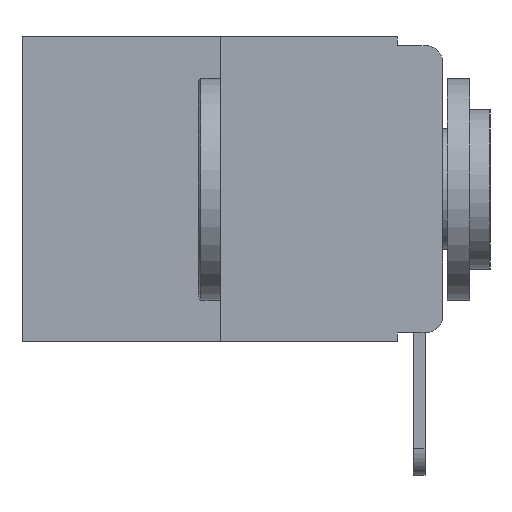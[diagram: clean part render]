
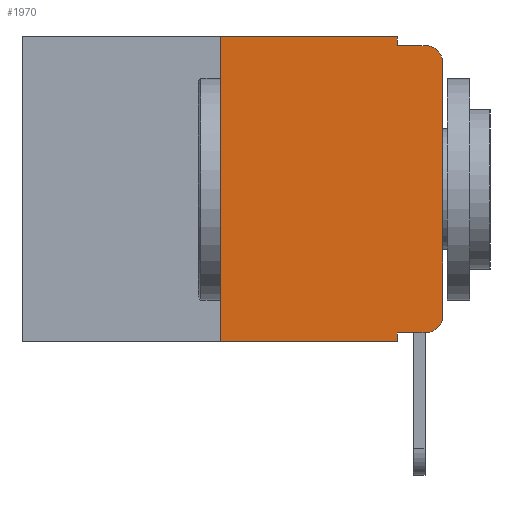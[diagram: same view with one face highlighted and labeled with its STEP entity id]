
A CAD part, left-side view. The second image highlights one B-rep face of the part: STEP entity #1970.
In plain terms, the highlighted planar face has unit normal (-1, 0, 0).
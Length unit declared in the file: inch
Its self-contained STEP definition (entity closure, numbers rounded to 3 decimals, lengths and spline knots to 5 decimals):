
#492 = CARTESIAN_POINT ( 'NONE',  ( 0., 0.051, -0.343 ) ) ;
#544 = VECTOR ( 'NONE', #5614, 39.37008 ) ;
#664 = FACE_OUTER_BOUND ( 'NONE', #9683, .T. ) ;
#940 = CARTESIAN_POINT ( 'NONE',  ( 0., 0.25, -0.343 ) ) ;
#1125 = VERTEX_POINT ( 'NONE', #9532 ) ;
#1679 = EDGE_CURVE ( 'NONE', #8181, #10054, #12038, .T. ) ;
#1754 = EDGE_CURVE ( 'NONE', #8181, #7487, #8797, .T. ) ;
#1970 = ADVANCED_FACE ( 'NONE', ( #664 ), #5951, .F. ) ;
#2189 = VERTEX_POINT ( 'NONE', #2217 ) ;
#2217 = CARTESIAN_POINT ( 'NONE',  ( 0., 0.02, -0.333 ) ) ;
#2447 = AXIS2_PLACEMENT_3D ( 'NONE', #4234, #10577, #5188 ) ;
#2629 = ORIENTED_EDGE ( 'NONE', *, *, #6933, .F. ) ;
#3120 = ORIENTED_EDGE ( 'NONE', *, *, #8857, .F. ) ;
#3358 = CARTESIAN_POINT ( 'NONE',  ( 0., 0.25, 0. ) ) ;
#3360 = LINE ( 'NONE', #7382, #544 ) ;
#3364 = CARTESIAN_POINT ( 'NONE',  ( 0., 0., -0.313 ) ) ;
#3394 = DIRECTION ( 'NONE',  ( 0., 0., 1. ) ) ;
#3437 = CIRCLE ( 'NONE', #7698, 0.02 ) ;
#3554 = LINE ( 'NONE', #5268, #8152 ) ;
#3770 = ORIENTED_EDGE ( 'NONE', *, *, #7630, .T. ) ;
#4046 = ORIENTED_EDGE ( 'NONE', *, *, #10227, .F. ) ;
#4164 = VECTOR ( 'NONE', #11022, 39.37008 ) ;
#4171 = CARTESIAN_POINT ( 'NONE',  ( 0., 0.051, -0.333 ) ) ;
#4234 = CARTESIAN_POINT ( 'NONE',  ( 0., 0.02, -0.03 ) ) ;
#4298 = CARTESIAN_POINT ( 'NONE',  ( 0., 0.051, -0.333 ) ) ;
#4332 = DIRECTION ( 'NONE',  ( 0., 0., -1. ) ) ;
#4460 = CARTESIAN_POINT ( 'NONE',  ( 0., 0.25, 0. ) ) ;
#4840 = VECTOR ( 'NONE', #3394, 39.37008 ) ;
#5188 = DIRECTION ( 'NONE',  ( 0., 0., -1. ) ) ;
#5268 = CARTESIAN_POINT ( 'NONE',  ( 0., 0.051, 0. ) ) ;
#5614 = DIRECTION ( 'NONE',  ( 0., -1., 0. ) ) ;
#5658 = CARTESIAN_POINT ( 'NONE',  ( 0., 0.473, 0. ) ) ;
#5678 = CARTESIAN_POINT ( 'NONE',  ( 0., 0.051, 0. ) ) ;
#5848 = DIRECTION ( 'NONE',  ( 1., 0., 0. ) ) ;
#5951 = PLANE ( 'NONE',  #8171 ) ;
#5974 = VECTOR ( 'NONE', #11630, 39.37008 ) ;
#5990 = DIRECTION ( 'NONE',  ( 0., 0., -1. ) ) ;
#6103 = CARTESIAN_POINT ( 'NONE',  ( 0., 0., -0.03 ) ) ;
#6165 = VECTOR ( 'NONE', #11073, 39.37008 ) ;
#6244 = CARTESIAN_POINT ( 'NONE',  ( 0., 0., 0. ) ) ;
#6442 = EDGE_CURVE ( 'NONE', #2189, #11906, #3437, .T. ) ;
#6578 = CARTESIAN_POINT ( 'NONE',  ( 0., 0.051, 0. ) ) ;
#6691 = VECTOR ( 'NONE', #11274, 39.37008 ) ;
#6828 = LINE ( 'NONE', #6244, #5974 ) ;
#6933 = EDGE_CURVE ( 'NONE', #10054, #7099, #10709, .T. ) ;
#7099 = VERTEX_POINT ( 'NONE', #6578 ) ;
#7195 = EDGE_CURVE ( 'NONE', #7099, #7977, #3554, .T. ) ;
#7382 = CARTESIAN_POINT ( 'NONE',  ( 0., 0.051, -0.01 ) ) ;
#7403 = CARTESIAN_POINT ( 'NONE',  ( 0., 0.473, -0.343 ) ) ;
#7487 = VERTEX_POINT ( 'NONE', #492 ) ;
#7630 = EDGE_CURVE ( 'NONE', #11870, #2189, #11404, .T. ) ;
#7698 = AXIS2_PLACEMENT_3D ( 'NONE', #10979, #10968, #10947 ) ;
#7977 = VERTEX_POINT ( 'NONE', #10114 ) ;
#8152 = VECTOR ( 'NONE', #4332, 39.37008 ) ;
#8171 = AXIS2_PLACEMENT_3D ( 'NONE', #5658, #5848, #5990 ) ;
#8181 = VERTEX_POINT ( 'NONE', #940 ) ;
#8297 = VECTOR ( 'NONE', #9332, 39.37008 ) ;
#8319 = VERTEX_POINT ( 'NONE', #6103 ) ;
#8797 = LINE ( 'NONE', #7403, #6691 ) ;
#8857 = EDGE_CURVE ( 'NONE', #11870, #7487, #11237, .T. ) ;
#9332 = DIRECTION ( 'NONE',  ( 0., -1., 0. ) ) ;
#9379 = CARTESIAN_POINT ( 'NONE',  ( 0., 0.473, 0. ) ) ;
#9532 = CARTESIAN_POINT ( 'NONE',  ( 0., 0.02, -0.01 ) ) ;
#9639 = ORIENTED_EDGE ( 'NONE', *, *, #11943, .T. ) ;
#9683 = EDGE_LOOP ( 'NONE', ( #9639, #12295, #4046, #11578, #2629, #11444, #12309, #3120, #3770, #11591 ) ) ;
#10054 = VERTEX_POINT ( 'NONE', #4460 ) ;
#10114 = CARTESIAN_POINT ( 'NONE',  ( 0., 0.051, -0.01 ) ) ;
#10227 = EDGE_CURVE ( 'NONE', #7977, #1125, #3360, .T. ) ;
#10577 = DIRECTION ( 'NONE',  ( -1., 0., 0. ) ) ;
#10601 = CIRCLE ( 'NONE', #2447, 0.02 ) ;
#10709 = LINE ( 'NONE', #9379, #8297 ) ;
#10947 = DIRECTION ( 'NONE',  ( 0., 0., -1. ) ) ;
#10968 = DIRECTION ( 'NONE',  ( -1., 0., 0. ) ) ;
#10979 = CARTESIAN_POINT ( 'NONE',  ( 0., 0.02, -0.313 ) ) ;
#11022 = DIRECTION ( 'NONE',  ( 0., -1., 0. ) ) ;
#11073 = DIRECTION ( 'NONE',  ( 0., 0., -1. ) ) ;
#11237 = LINE ( 'NONE', #5678, #6165 ) ;
#11274 = DIRECTION ( 'NONE',  ( 0., -1., 0. ) ) ;
#11404 = LINE ( 'NONE', #4171, #4164 ) ;
#11444 = ORIENTED_EDGE ( 'NONE', *, *, #1679, .F. ) ;
#11578 = ORIENTED_EDGE ( 'NONE', *, *, #7195, .F. ) ;
#11591 = ORIENTED_EDGE ( 'NONE', *, *, #6442, .T. ) ;
#11630 = DIRECTION ( 'NONE',  ( 0., 0., 1. ) ) ;
#11870 = VERTEX_POINT ( 'NONE', #4298 ) ;
#11906 = VERTEX_POINT ( 'NONE', #3364 ) ;
#11943 = EDGE_CURVE ( 'NONE', #11906, #8319, #6828, .T. ) ;
#12038 = LINE ( 'NONE', #3358, #4840 ) ;
#12181 = EDGE_CURVE ( 'NONE', #8319, #1125, #10601, .T. ) ;
#12295 = ORIENTED_EDGE ( 'NONE', *, *, #12181, .T. ) ;
#12309 = ORIENTED_EDGE ( 'NONE', *, *, #1754, .T. ) ;
